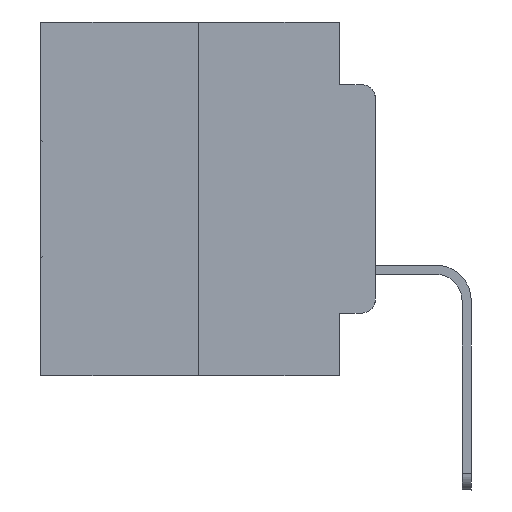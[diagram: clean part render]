
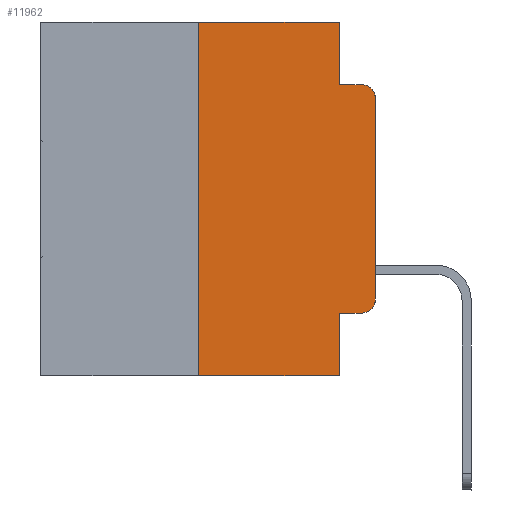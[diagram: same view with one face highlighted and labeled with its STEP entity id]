
A CAD part, left-side view. The second image highlights one B-rep face of the part: STEP entity #11962.
In plain terms, the highlighted planar face has unit normal (-1, 0, 0).
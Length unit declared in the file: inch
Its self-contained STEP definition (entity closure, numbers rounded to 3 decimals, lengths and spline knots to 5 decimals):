
#464 = DIRECTION ( 'NONE',  ( 0., 0., 1. ) ) ;
#823 = CARTESIAN_POINT ( 'NONE',  ( 0., 0.25, -0.5 ) ) ;
#1192 = DIRECTION ( 'NONE',  ( 0., 0., -1. ) ) ;
#1816 = CARTESIAN_POINT ( 'NONE',  ( 0., 0.02, -0.1085 ) ) ;
#2934 = VERTEX_POINT ( 'NONE', #5184 ) ;
#3481 = CARTESIAN_POINT ( 'NONE',  ( 0., 0.473, -0.5 ) ) ;
#3638 = ORIENTED_EDGE ( 'NONE', *, *, #9325, .F. ) ;
#3768 = EDGE_CURVE ( 'NONE', #20404, #24811, #10581, .T. ) ;
#3880 = VECTOR ( 'NONE', #11698, 39.37008 ) ;
#4108 = DIRECTION ( 'NONE',  ( 0., 0., -1. ) ) ;
#4147 = DIRECTION ( 'NONE',  ( -1., 0., 0. ) ) ;
#4628 = VERTEX_POINT ( 'NONE', #17070 ) ;
#4990 = EDGE_CURVE ( 'NONE', #13117, #8996, #28199, .T. ) ;
#5184 = CARTESIAN_POINT ( 'NONE',  ( 0., 0., -0.3915 ) ) ;
#6797 = CARTESIAN_POINT ( 'NONE',  ( 0., 0., 0. ) ) ;
#7316 = CARTESIAN_POINT ( 'NONE',  ( 0., 0.051, -0.4115 ) ) ;
#7828 = ORIENTED_EDGE ( 'NONE', *, *, #8429, .F. ) ;
#8087 = ORIENTED_EDGE ( 'NONE', *, *, #15684, .T. ) ;
#8429 = EDGE_CURVE ( 'NONE', #20404, #17805, #24722, .T. ) ;
#8597 = EDGE_CURVE ( 'NONE', #17805, #10624, #11497, .T. ) ;
#8685 = DIRECTION ( 'NONE',  ( 0., 0., -1. ) ) ;
#8962 = VECTOR ( 'NONE', #22331, 39.37008 ) ;
#8994 = VECTOR ( 'NONE', #1192, 39.37008 ) ;
#8996 = VERTEX_POINT ( 'NONE', #26647 ) ;
#9242 = AXIS2_PLACEMENT_3D ( 'NONE', #11711, #16092, #9354 ) ;
#9266 = AXIS2_PLACEMENT_3D ( 'NONE', #1816, #4147, #8685 ) ;
#9325 = EDGE_CURVE ( 'NONE', #10624, #13117, #25352, .T. ) ;
#9354 = DIRECTION ( 'NONE',  ( 0., 0., -1. ) ) ;
#9771 = CARTESIAN_POINT ( 'NONE',  ( 0., 0.473, 0. ) ) ;
#10010 = CARTESIAN_POINT ( 'NONE',  ( 0., 0.02, -0.3915 ) ) ;
#10114 = CARTESIAN_POINT ( 'NONE',  ( 0., 0.051, 0. ) ) ;
#10581 = LINE ( 'NONE', #3481, #10909 ) ;
#10624 = VERTEX_POINT ( 'NONE', #10114 ) ;
#10909 = VECTOR ( 'NONE', #14748, 39.37008 ) ;
#10975 = EDGE_LOOP ( 'NONE', ( #19846, #28730, #17374, #3638, #26431, #7828, #17132, #15850, #17961, #8087 ) ) ;
#11159 = VECTOR ( 'NONE', #16490, 39.37008 ) ;
#11497 = LINE ( 'NONE', #9771, #11159 ) ;
#11698 = DIRECTION ( 'NONE',  ( 0., -1., 0. ) ) ;
#11711 = CARTESIAN_POINT ( 'NONE',  ( 0., 0.473, 0. ) ) ;
#11962 = ADVANCED_FACE ( 'NONE', ( #28643 ), #22970, .F. ) ;
#12507 = EDGE_CURVE ( 'NONE', #17221, #24811, #22109, .T. ) ;
#13117 = VERTEX_POINT ( 'NONE', #20603 ) ;
#13273 = VECTOR ( 'NONE', #18431, 39.37008 ) ;
#13871 = CARTESIAN_POINT ( 'NONE',  ( 0., 0.25, 0. ) ) ;
#14669 = DIRECTION ( 'NONE',  ( 0., 0., -1. ) ) ;
#14748 = DIRECTION ( 'NONE',  ( 0., -1., 0. ) ) ;
#15235 = LINE ( 'NONE', #6797, #8962 ) ;
#15684 = EDGE_CURVE ( 'NONE', #4628, #2934, #23328, .T. ) ;
#15850 = ORIENTED_EDGE ( 'NONE', *, *, #12507, .F. ) ;
#15862 = EDGE_CURVE ( 'NONE', #2934, #16907, #15235, .T. ) ;
#16092 = DIRECTION ( 'NONE',  ( 1., 0., 0. ) ) ;
#16362 = CARTESIAN_POINT ( 'NONE',  ( 0., 0.051, -0.0885 ) ) ;
#16490 = DIRECTION ( 'NONE',  ( 0., -1., 0. ) ) ;
#16542 = DIRECTION ( 'NONE',  ( -1., 0., 0. ) ) ;
#16573 = CARTESIAN_POINT ( 'NONE',  ( 0., 0., -0.1085 ) ) ;
#16907 = VERTEX_POINT ( 'NONE', #16573 ) ;
#17031 = CARTESIAN_POINT ( 'NONE',  ( 0., 0.051, 0. ) ) ;
#17070 = CARTESIAN_POINT ( 'NONE',  ( 0., 0.02, -0.4115 ) ) ;
#17132 = ORIENTED_EDGE ( 'NONE', *, *, #3768, .T. ) ;
#17221 = VERTEX_POINT ( 'NONE', #22350 ) ;
#17374 = ORIENTED_EDGE ( 'NONE', *, *, #4990, .F. ) ;
#17805 = VERTEX_POINT ( 'NONE', #21766 ) ;
#17961 = ORIENTED_EDGE ( 'NONE', *, *, #25756, .T. ) ;
#18313 = EDGE_CURVE ( 'NONE', #16907, #8996, #22033, .T. ) ;
#18431 = DIRECTION ( 'NONE',  ( 0., -1., 0. ) ) ;
#18856 = VECTOR ( 'NONE', #464, 39.37008 ) ;
#19201 = LINE ( 'NONE', #7316, #13273 ) ;
#19846 = ORIENTED_EDGE ( 'NONE', *, *, #15862, .T. ) ;
#19942 = CARTESIAN_POINT ( 'NONE',  ( 0., 0.051, 0. ) ) ;
#20404 = VERTEX_POINT ( 'NONE', #823 ) ;
#20603 = CARTESIAN_POINT ( 'NONE',  ( 0., 0.051, -0.0885 ) ) ;
#21702 = CARTESIAN_POINT ( 'NONE',  ( 0., 0.051, -0.5 ) ) ;
#21766 = CARTESIAN_POINT ( 'NONE',  ( 0., 0.25, 0. ) ) ;
#22033 = CIRCLE ( 'NONE', #9266, 0.02 ) ;
#22109 = LINE ( 'NONE', #19942, #26254 ) ;
#22331 = DIRECTION ( 'NONE',  ( 0., 0., 1. ) ) ;
#22350 = CARTESIAN_POINT ( 'NONE',  ( 0., 0.051, -0.4115 ) ) ;
#22970 = PLANE ( 'NONE',  #9242 ) ;
#23328 = CIRCLE ( 'NONE', #27000, 0.02 ) ;
#24722 = LINE ( 'NONE', #13871, #18856 ) ;
#24811 = VERTEX_POINT ( 'NONE', #21702 ) ;
#25352 = LINE ( 'NONE', #17031, #8994 ) ;
#25756 = EDGE_CURVE ( 'NONE', #17221, #4628, #19201, .T. ) ;
#26254 = VECTOR ( 'NONE', #4108, 39.37008 ) ;
#26431 = ORIENTED_EDGE ( 'NONE', *, *, #8597, .F. ) ;
#26647 = CARTESIAN_POINT ( 'NONE',  ( 0., 0.02, -0.0885 ) ) ;
#27000 = AXIS2_PLACEMENT_3D ( 'NONE', #10010, #16542, #14669 ) ;
#28199 = LINE ( 'NONE', #16362, #3880 ) ;
#28643 = FACE_OUTER_BOUND ( 'NONE', #10975, .T. ) ;
#28730 = ORIENTED_EDGE ( 'NONE', *, *, #18313, .T. ) ;
